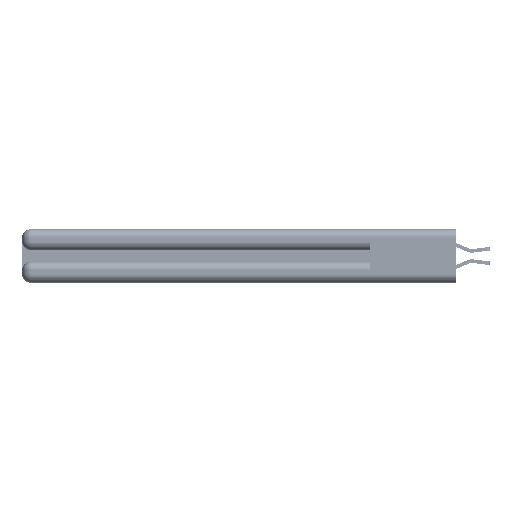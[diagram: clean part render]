
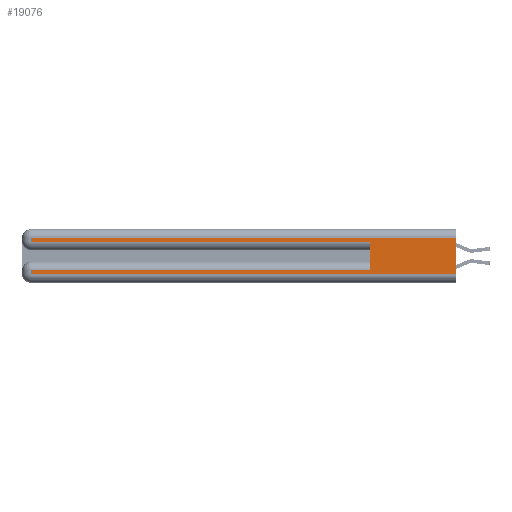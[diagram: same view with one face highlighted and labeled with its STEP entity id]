
A CAD part, left-side view. The second image highlights one B-rep face of the part: STEP entity #19076.
In plain terms, the highlighted planar face has unit normal (-1, 0, 0).
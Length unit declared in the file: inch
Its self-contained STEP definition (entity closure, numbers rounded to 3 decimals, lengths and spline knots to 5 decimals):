
#408 = LINE ( 'NONE', #8766, #16607 ) ;
#657 = VECTOR ( 'NONE', #19794, 39.37008 ) ;
#796 = VERTEX_POINT ( 'NONE', #37109 ) ;
#825 = CARTESIAN_POINT ( 'NONE',  ( 0., 0., 0.285 ) ) ;
#4924 = DIRECTION ( 'NONE',  ( 0., 1., 0. ) ) ;
#4967 = CARTESIAN_POINT ( 'NONE',  ( 0., 2.94, 0.285 ) ) ;
#5089 = CARTESIAN_POINT ( 'NONE',  ( 0., 0., 0.06 ) ) ;
#6292 = CARTESIAN_POINT ( 'NONE',  ( 0., 2.94, 0.085 ) ) ;
#7358 = DIRECTION ( 'NONE',  ( 0., 1., 0. ) ) ;
#7653 = LINE ( 'NONE', #18024, #23857 ) ;
#8235 = VERTEX_POINT ( 'NONE', #20716 ) ;
#8766 = CARTESIAN_POINT ( 'NONE',  ( 0., 0., 0.31 ) ) ;
#8999 = DIRECTION ( 'NONE',  ( 0., -1., 0. ) ) ;
#9334 = VECTOR ( 'NONE', #39876, 39.37008 ) ;
#11758 = CARTESIAN_POINT ( 'NONE',  ( 0., 2.94, 0.37 ) ) ;
#12420 = EDGE_CURVE ( 'NONE', #30606, #15487, #23018, .T. ) ;
#12691 = ORIENTED_EDGE ( 'NONE', *, *, #27556, .T. ) ;
#13074 = ORIENTED_EDGE ( 'NONE', *, *, #24400, .F. ) ;
#15395 = DIRECTION ( 'NONE',  ( 1., 0., 0. ) ) ;
#15487 = VERTEX_POINT ( 'NONE', #4967 ) ;
#15529 = VERTEX_POINT ( 'NONE', #48817 ) ;
#15655 = LINE ( 'NONE', #39332, #39264 ) ;
#15819 = ORIENTED_EDGE ( 'NONE', *, *, #19512, .T. ) ;
#15876 = VERTEX_POINT ( 'NONE', #40043 ) ;
#16607 = VECTOR ( 'NONE', #4924, 39.37008 ) ;
#17855 = DIRECTION ( 'NONE',  ( 0., 0., -1. ) ) ;
#18024 = CARTESIAN_POINT ( 'NONE',  ( 0., 0., 0.37 ) ) ;
#18358 = ORIENTED_EDGE ( 'NONE', *, *, #21520, .F. ) ;
#18670 = EDGE_CURVE ( 'NONE', #15487, #8235, #26294, .T. ) ;
#19076 = ADVANCED_FACE ( 'NONE', ( #22588 ), #23752, .F. ) ;
#19512 = EDGE_CURVE ( 'NONE', #796, #32534, #15655, .T. ) ;
#19794 = DIRECTION ( 'NONE',  ( 0., 0., -1. ) ) ;
#20716 = CARTESIAN_POINT ( 'NONE',  ( 0., 0.6, 0.285 ) ) ;
#21520 = EDGE_CURVE ( 'NONE', #796, #8235, #47122, .T. ) ;
#22493 = EDGE_CURVE ( 'NONE', #15876, #30606, #408, .T. ) ;
#22588 = FACE_OUTER_BOUND ( 'NONE', #47097, .T. ) ;
#23018 = LINE ( 'NONE', #28264, #9334 ) ;
#23552 = DIRECTION ( 'NONE',  ( 0., 0., 1. ) ) ;
#23752 = PLANE ( 'NONE',  #45068 ) ;
#23857 = VECTOR ( 'NONE', #17855, 39.37008 ) ;
#24400 = EDGE_CURVE ( 'NONE', #15876, #26372, #7653, .T. ) ;
#26294 = LINE ( 'NONE', #825, #28830 ) ;
#26372 = VERTEX_POINT ( 'NONE', #47964 ) ;
#27556 = EDGE_CURVE ( 'NONE', #15529, #26372, #42252, .T. ) ;
#28264 = CARTESIAN_POINT ( 'NONE',  ( 0., 2.94, 0.37 ) ) ;
#28830 = VECTOR ( 'NONE', #8999, 39.37008 ) ;
#30257 = CARTESIAN_POINT ( 'NONE',  ( 0., 2.94, 0.31 ) ) ;
#30606 = VERTEX_POINT ( 'NONE', #30257 ) ;
#32534 = VERTEX_POINT ( 'NONE', #6292 ) ;
#33440 = VECTOR ( 'NONE', #23552, 39.37008 ) ;
#33621 = LINE ( 'NONE', #11758, #657 ) ;
#35680 = CARTESIAN_POINT ( 'NONE',  ( 0., 0.6, 0.145 ) ) ;
#37109 = CARTESIAN_POINT ( 'NONE',  ( 0., 0.6, 0.085 ) ) ;
#38686 = ORIENTED_EDGE ( 'NONE', *, *, #40166, .T. ) ;
#39264 = VECTOR ( 'NONE', #7358, 39.37008 ) ;
#39306 = ORIENTED_EDGE ( 'NONE', *, *, #18670, .T. ) ;
#39332 = CARTESIAN_POINT ( 'NONE',  ( 0., 0., 0.085 ) ) ;
#39876 = DIRECTION ( 'NONE',  ( 0., 0., -1. ) ) ;
#40043 = CARTESIAN_POINT ( 'NONE',  ( 0., 0., 0.31 ) ) ;
#40166 = EDGE_CURVE ( 'NONE', #32534, #15529, #33621, .T. ) ;
#41776 = ORIENTED_EDGE ( 'NONE', *, *, #12420, .T. ) ;
#42252 = LINE ( 'NONE', #5089, #50920 ) ;
#43350 = DIRECTION ( 'NONE',  ( 0., 0., -1. ) ) ;
#44585 = DIRECTION ( 'NONE',  ( 0., -1., 0. ) ) ;
#45068 = AXIS2_PLACEMENT_3D ( 'NONE', #51190, #15395, #43350 ) ;
#47097 = EDGE_LOOP ( 'NONE', ( #13074, #48548, #41776, #39306, #18358, #15819, #38686, #12691 ) ) ;
#47122 = LINE ( 'NONE', #35680, #33440 ) ;
#47964 = CARTESIAN_POINT ( 'NONE',  ( 0., 0., 0.06 ) ) ;
#48548 = ORIENTED_EDGE ( 'NONE', *, *, #22493, .T. ) ;
#48817 = CARTESIAN_POINT ( 'NONE',  ( 0., 2.94, 0.06 ) ) ;
#50920 = VECTOR ( 'NONE', #44585, 39.37008 ) ;
#51190 = CARTESIAN_POINT ( 'NONE',  ( 0., 0., 0.37 ) ) ;
